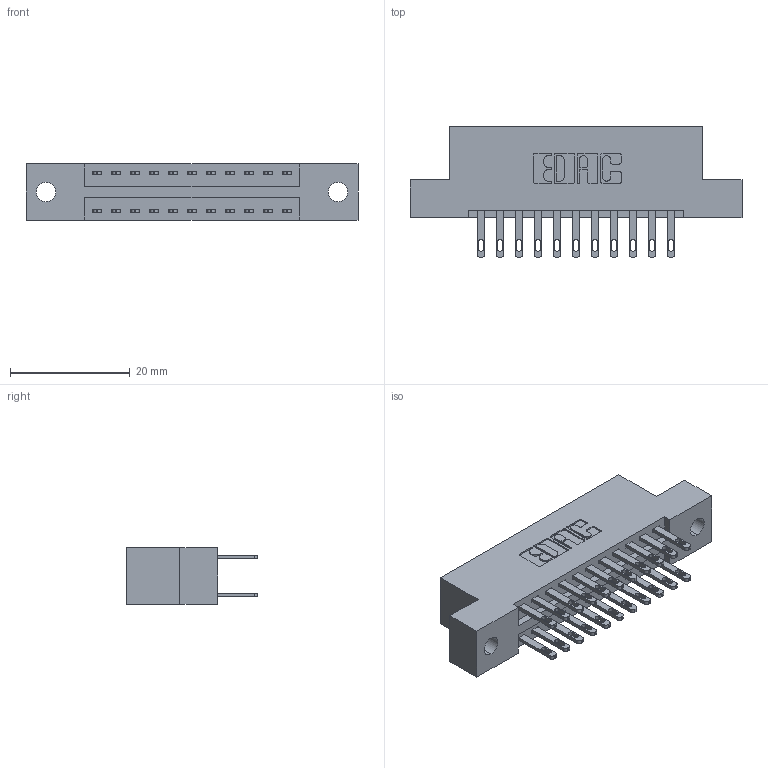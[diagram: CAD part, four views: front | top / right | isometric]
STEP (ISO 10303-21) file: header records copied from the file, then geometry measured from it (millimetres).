
FILE_DESCRIPTION (( 'STEP AP203' ), '1' );
FILE_NAME ('346-022-500-202.STEP', '2022-05-18T20:24:45', ( '' ), ( '' ), 'SwSTEP 2.0', 'SolidWorks 2020', '' );
FILE_SCHEMA (( 'CONFIG_CONTROL_DESIGN' ));
Length unit declared in the file: inch
Products named in the file (3): 345-292-001_345-293-100; 346-022-500-202; 346 Part_Flush Mounting Lugs - 0.128 Dia
Assembly tree (23 placements, depth 2):
  346-022-500-202
    346 Part_Flush Mounting Lugs - 0.128 Dia
    345-292-001_345-293-100  x22
Bounding box: 55.5 x 21.84 x 9.4 mm (x, y, z)
Volume: 5201.6 mm3; surface area: 6623.7 mm2
Topology: 23 solids, 23 shells, 1178 faces, 3563 edges, 2374 vertices
Faces by surface type: plane 714, cylinder 464
Entity records: 11285 total; most frequent: CARTESIAN_POINT 1900, ORIENTED_EDGE 1834, DIRECTION 1729, EDGE_CURVE 917, LINE 737, VECTOR 737, VERTEX_POINT 610, AXIS2_PLACEMENT_3D 496
